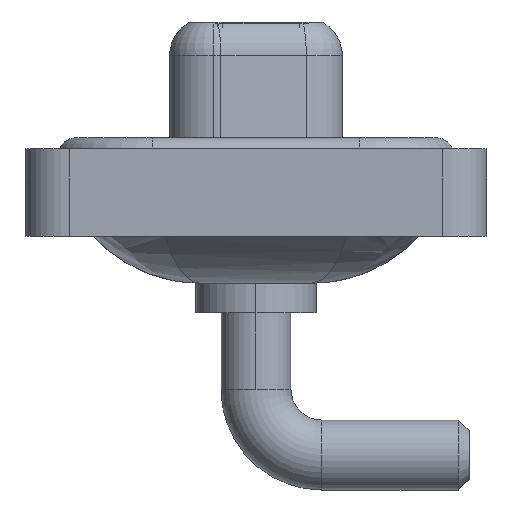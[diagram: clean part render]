
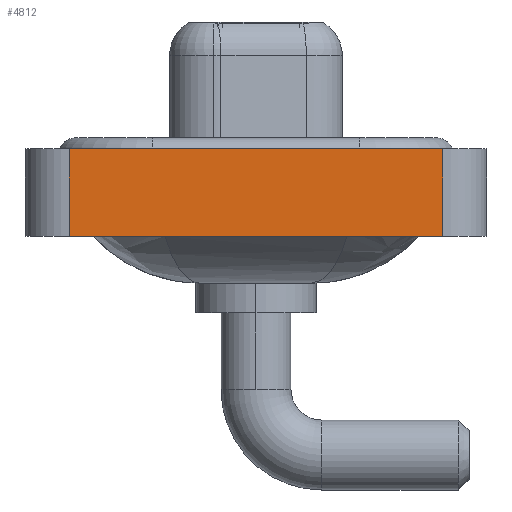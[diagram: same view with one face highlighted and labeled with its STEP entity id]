
A CAD part, left-side view. The second image highlights one B-rep face of the part: STEP entity #4812.
In plain terms, the highlighted planar face has unit normal (-1, 0, 0).
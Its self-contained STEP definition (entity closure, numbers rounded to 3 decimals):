
#433 = LINE ( 'NONE', #4253, #11070 ) ;
#917 = CARTESIAN_POINT ( 'NONE',  ( -7.35, 8.55, -3.6 ) ) ;
#1322 = EDGE_CURVE ( 'NONE', #11967, #8490, #15747, .T. ) ;
#1387 = CARTESIAN_POINT ( 'NONE',  ( -7.35, -8.55, -3.6 ) ) ;
#1446 = EDGE_CURVE ( 'NONE', #11967, #5235, #433, .T. ) ;
#1773 = EDGE_CURVE ( 'NONE', #8490, #9150, #6287, .T. ) ;
#2529 = AXIS2_PLACEMENT_3D ( 'NONE', #3256, #13792, #10076 ) ;
#2616 = DIRECTION ( 'NONE',  ( 0., 0., 1. ) ) ;
#3256 = CARTESIAN_POINT ( 'NONE',  ( -7.35, -8.55, -3.6 ) ) ;
#4006 = ORIENTED_EDGE ( 'NONE', *, *, #1773, .F. ) ;
#4253 = CARTESIAN_POINT ( 'NONE',  ( -7.35, -8.55, -3.6 ) ) ;
#4599 = CARTESIAN_POINT ( 'NONE',  ( -7.35, 8.55, 0.4 ) ) ;
#4812 = ADVANCED_FACE ( 'NONE', ( #9590 ), #14649, .T. ) ;
#5235 = VERTEX_POINT ( 'NONE', #1387 ) ;
#5462 = VECTOR ( 'NONE', #9599, 1000. ) ;
#5479 = CARTESIAN_POINT ( 'NONE',  ( -7.35, -8.55, 0.4 ) ) ;
#6287 = LINE ( 'NONE', #12774, #16091 ) ;
#8426 = ORIENTED_EDGE ( 'NONE', *, *, #1322, .F. ) ;
#8469 = ORIENTED_EDGE ( 'NONE', *, *, #1446, .T. ) ;
#8490 = VERTEX_POINT ( 'NONE', #4599 ) ;
#8814 = DIRECTION ( 'NONE',  ( 0., -1., 0. ) ) ;
#8865 = CARTESIAN_POINT ( 'NONE',  ( -7.35, -8.55, -3.6 ) ) ;
#9150 = VERTEX_POINT ( 'NONE', #5479 ) ;
#9434 = CARTESIAN_POINT ( 'NONE',  ( -7.35, 8.55, -3.6 ) ) ;
#9590 = FACE_OUTER_BOUND ( 'NONE', #15482, .T. ) ;
#9599 = DIRECTION ( 'NONE',  ( 0., 0., 1. ) ) ;
#9900 = EDGE_CURVE ( 'NONE', #5235, #9150, #12917, .T. ) ;
#10076 = DIRECTION ( 'NONE',  ( 0., 0., 1. ) ) ;
#10349 = ORIENTED_EDGE ( 'NONE', *, *, #9900, .T. ) ;
#11070 = VECTOR ( 'NONE', #14399, 1000. ) ;
#11967 = VERTEX_POINT ( 'NONE', #917 ) ;
#12037 = VECTOR ( 'NONE', #2616, 1000. ) ;
#12774 = CARTESIAN_POINT ( 'NONE',  ( -7.35, -8.55, 0.4 ) ) ;
#12917 = LINE ( 'NONE', #8865, #12037 ) ;
#13792 = DIRECTION ( 'NONE',  ( -1., 0., 0. ) ) ;
#14399 = DIRECTION ( 'NONE',  ( 0., -1., 0. ) ) ;
#14649 = PLANE ( 'NONE',  #2529 ) ;
#15482 = EDGE_LOOP ( 'NONE', ( #10349, #4006, #8426, #8469 ) ) ;
#15747 = LINE ( 'NONE', #9434, #5462 ) ;
#16091 = VECTOR ( 'NONE', #8814, 1000. ) ;
